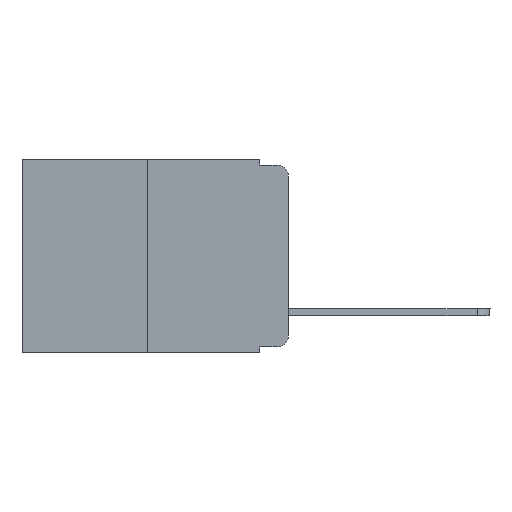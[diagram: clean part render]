
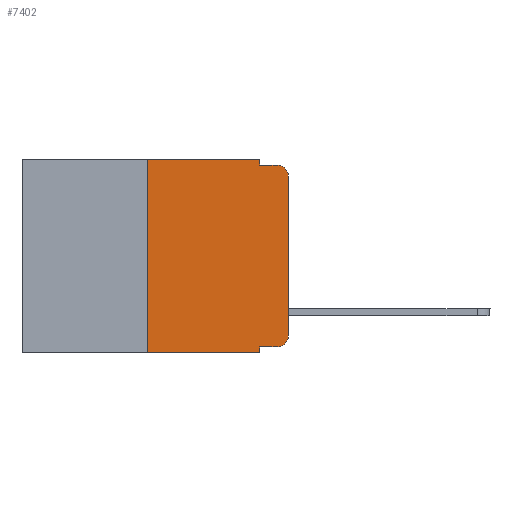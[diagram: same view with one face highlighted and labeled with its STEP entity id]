
A CAD part, left-side view. The second image highlights one B-rep face of the part: STEP entity #7402.
In plain terms, the highlighted planar face has unit normal (-1, 0, 0).
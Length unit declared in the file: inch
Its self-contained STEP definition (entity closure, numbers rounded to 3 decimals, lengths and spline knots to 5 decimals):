
#43 = EDGE_CURVE ( 'NONE', #2771, #17003, #5073, .T. ) ;
#297 = LINE ( 'NONE', #14133, #3050 ) ;
#363 = CARTESIAN_POINT ( 'NONE',  ( 0., 0.051, 0. ) ) ;
#372 = VERTEX_POINT ( 'NONE', #19795 ) ;
#681 = ORIENTED_EDGE ( 'NONE', *, *, #10820, .F. ) ;
#908 = DIRECTION ( 'NONE',  ( 0., 0., 1. ) ) ;
#1180 = ORIENTED_EDGE ( 'NONE', *, *, #12720, .T. ) ;
#1209 = LINE ( 'NONE', #5825, #10590 ) ;
#1349 = DIRECTION ( 'NONE',  ( 0., -1., 0. ) ) ;
#1656 = EDGE_CURVE ( 'NONE', #1771, #7334, #2343, .T. ) ;
#1771 = VERTEX_POINT ( 'NONE', #10148 ) ;
#2038 = VERTEX_POINT ( 'NONE', #13016 ) ;
#2343 = LINE ( 'NONE', #14372, #6940 ) ;
#2717 = ORIENTED_EDGE ( 'NONE', *, *, #11670, .T. ) ;
#2725 = VECTOR ( 'NONE', #4521, 39.37008 ) ;
#2771 = VERTEX_POINT ( 'NONE', #10152 ) ;
#2999 = PLANE ( 'NONE',  #8249 ) ;
#3050 = VECTOR ( 'NONE', #6714, 39.37008 ) ;
#3156 = CARTESIAN_POINT ( 'NONE',  ( 0., 0.051, -0.333 ) ) ;
#3179 = LINE ( 'NONE', #363, #12967 ) ;
#4228 = CARTESIAN_POINT ( 'NONE',  ( 0., 0., -0.03 ) ) ;
#4297 = DIRECTION ( 'NONE',  ( 0., 0., -1. ) ) ;
#4368 = ORIENTED_EDGE ( 'NONE', *, *, #14026, .T. ) ;
#4415 = CARTESIAN_POINT ( 'NONE',  ( 0., 0.473, -0.343 ) ) ;
#4521 = DIRECTION ( 'NONE',  ( 0., -1., 0. ) ) ;
#5073 = LINE ( 'NONE', #12490, #13193 ) ;
#5794 = ORIENTED_EDGE ( 'NONE', *, *, #13876, .T. ) ;
#5825 = CARTESIAN_POINT ( 'NONE',  ( 0., 0.051, -0.01 ) ) ;
#5996 = ORIENTED_EDGE ( 'NONE', *, *, #43, .F. ) ;
#6309 = CARTESIAN_POINT ( 'NONE',  ( 0., 0.02, -0.03 ) ) ;
#6371 = DIRECTION ( 'NONE',  ( 0., 0., -1. ) ) ;
#6594 = VERTEX_POINT ( 'NONE', #3156 ) ;
#6714 = DIRECTION ( 'NONE',  ( 0., -1., 0. ) ) ;
#6940 = VECTOR ( 'NONE', #17875, 39.37008 ) ;
#6990 = CIRCLE ( 'NONE', #19171, 0.02 ) ;
#7250 = CARTESIAN_POINT ( 'NONE',  ( 0., 0.02, -0.333 ) ) ;
#7334 = VERTEX_POINT ( 'NONE', #14921 ) ;
#7402 = ADVANCED_FACE ( 'NONE', ( #13917 ), #2999, .F. ) ;
#7551 = CARTESIAN_POINT ( 'NONE',  ( 0., 0.051, -0.343 ) ) ;
#7594 = AXIS2_PLACEMENT_3D ( 'NONE', #6309, #12425, #13828 ) ;
#7803 = DIRECTION ( 'NONE',  ( 0., 0., -1. ) ) ;
#8029 = CARTESIAN_POINT ( 'NONE',  ( 0., 0.051, -0.01 ) ) ;
#8249 = AXIS2_PLACEMENT_3D ( 'NONE', #12318, #14729, #7803 ) ;
#8429 = LINE ( 'NONE', #8720, #19515 ) ;
#8720 = CARTESIAN_POINT ( 'NONE',  ( 0., 0., 0. ) ) ;
#8749 = EDGE_CURVE ( 'NONE', #11244, #372, #12402, .T. ) ;
#8935 = VECTOR ( 'NONE', #1349, 39.37008 ) ;
#9453 = VERTEX_POINT ( 'NONE', #7250 ) ;
#9535 = VERTEX_POINT ( 'NONE', #7551 ) ;
#10148 = CARTESIAN_POINT ( 'NONE',  ( 0., 0.25, -0.343 ) ) ;
#10152 = CARTESIAN_POINT ( 'NONE',  ( 0., 0.051, 0. ) ) ;
#10590 = VECTOR ( 'NONE', #16648, 39.37008 ) ;
#10820 = EDGE_CURVE ( 'NONE', #7334, #2771, #15268, .T. ) ;
#11244 = VERTEX_POINT ( 'NONE', #4228 ) ;
#11670 = EDGE_CURVE ( 'NONE', #9453, #2038, #6990, .T. ) ;
#12318 = CARTESIAN_POINT ( 'NONE',  ( 0., 0.473, 0. ) ) ;
#12402 = CIRCLE ( 'NONE', #7594, 0.02 ) ;
#12425 = DIRECTION ( 'NONE',  ( -1., 0., 0. ) ) ;
#12490 = CARTESIAN_POINT ( 'NONE',  ( 0., 0.051, 0. ) ) ;
#12720 = EDGE_CURVE ( 'NONE', #2038, #11244, #8429, .T. ) ;
#12967 = VECTOR ( 'NONE', #13996, 39.37008 ) ;
#13016 = CARTESIAN_POINT ( 'NONE',  ( 0., 0., -0.313 ) ) ;
#13193 = VECTOR ( 'NONE', #6371, 39.37008 ) ;
#13433 = EDGE_CURVE ( 'NONE', #6594, #9535, #3179, .T. ) ;
#13828 = DIRECTION ( 'NONE',  ( 0., 0., -1. ) ) ;
#13876 = EDGE_CURVE ( 'NONE', #1771, #9535, #18353, .T. ) ;
#13917 = FACE_OUTER_BOUND ( 'NONE', #16818, .T. ) ;
#13996 = DIRECTION ( 'NONE',  ( 0., 0., -1. ) ) ;
#14026 = EDGE_CURVE ( 'NONE', #6594, #9453, #297, .T. ) ;
#14064 = ORIENTED_EDGE ( 'NONE', *, *, #16875, .F. ) ;
#14133 = CARTESIAN_POINT ( 'NONE',  ( 0., 0.051, -0.333 ) ) ;
#14372 = CARTESIAN_POINT ( 'NONE',  ( 0., 0.25, 0. ) ) ;
#14486 = ORIENTED_EDGE ( 'NONE', *, *, #1656, .F. ) ;
#14579 = ORIENTED_EDGE ( 'NONE', *, *, #13433, .F. ) ;
#14729 = DIRECTION ( 'NONE',  ( 1., 0., 0. ) ) ;
#14921 = CARTESIAN_POINT ( 'NONE',  ( 0., 0.25, 0. ) ) ;
#15163 = CARTESIAN_POINT ( 'NONE',  ( 0., 0.473, 0. ) ) ;
#15268 = LINE ( 'NONE', #15163, #8935 ) ;
#15709 = ORIENTED_EDGE ( 'NONE', *, *, #8749, .T. ) ;
#16648 = DIRECTION ( 'NONE',  ( 0., -1., 0. ) ) ;
#16818 = EDGE_LOOP ( 'NONE', ( #1180, #15709, #14064, #5996, #681, #14486, #5794, #14579, #4368, #2717 ) ) ;
#16875 = EDGE_CURVE ( 'NONE', #17003, #372, #1209, .T. ) ;
#17003 = VERTEX_POINT ( 'NONE', #8029 ) ;
#17875 = DIRECTION ( 'NONE',  ( 0., 0., 1. ) ) ;
#18134 = CARTESIAN_POINT ( 'NONE',  ( 0., 0.02, -0.313 ) ) ;
#18353 = LINE ( 'NONE', #4415, #2725 ) ;
#19171 = AXIS2_PLACEMENT_3D ( 'NONE', #18134, #19745, #4297 ) ;
#19515 = VECTOR ( 'NONE', #908, 39.37008 ) ;
#19745 = DIRECTION ( 'NONE',  ( -1., 0., 0. ) ) ;
#19795 = CARTESIAN_POINT ( 'NONE',  ( 0., 0.02, -0.01 ) ) ;
